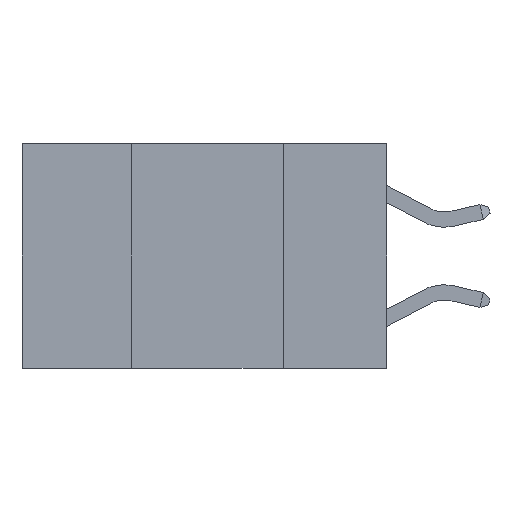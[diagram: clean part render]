
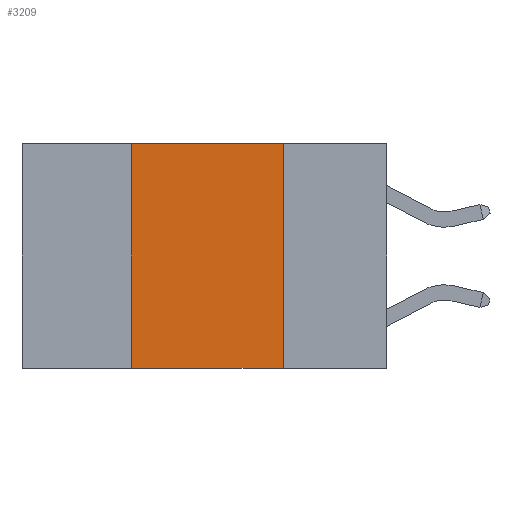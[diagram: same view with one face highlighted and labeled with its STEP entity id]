
A CAD part, left-side view. The second image highlights one B-rep face of the part: STEP entity #3209.
In plain terms, the highlighted planar face has unit normal (-1, 0, 0).
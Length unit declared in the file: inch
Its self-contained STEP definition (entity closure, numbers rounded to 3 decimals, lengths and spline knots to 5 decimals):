
#178 = LINE ( 'NONE', #4160, #14691 ) ;
#516 = EDGE_CURVE ( 'NONE', #11932, #4437, #6694, .T. ) ;
#741 = CARTESIAN_POINT ( 'NONE',  ( 0., 0.17, 0. ) ) ;
#879 = LINE ( 'NONE', #4568, #3562 ) ;
#1176 = CARTESIAN_POINT ( 'NONE',  ( 0., 0.42, 0. ) ) ;
#2120 = DIRECTION ( 'NONE',  ( 0., -1., 0. ) ) ;
#2227 = EDGE_CURVE ( 'NONE', #11945, #11932, #8086, .T. ) ;
#2247 = EDGE_CURVE ( 'NONE', #4437, #12415, #879, .T. ) ;
#2330 = EDGE_CURVE ( 'NONE', #11945, #12415, #178, .T. ) ;
#2618 = DIRECTION ( 'NONE',  ( 0., 0., 1. ) ) ;
#3209 = ADVANCED_FACE ( 'NONE', ( #7870 ), #11098, .F. ) ;
#3328 = CARTESIAN_POINT ( 'NONE',  ( 0., 0.17, -0.37 ) ) ;
#3562 = VECTOR ( 'NONE', #4903, 39.37008 ) ;
#4160 = CARTESIAN_POINT ( 'NONE',  ( 0., 0.6, -0.37 ) ) ;
#4239 = DIRECTION ( 'NONE',  ( 1., 0., 0. ) ) ;
#4437 = VERTEX_POINT ( 'NONE', #741 ) ;
#4568 = CARTESIAN_POINT ( 'NONE',  ( 0., 0.17, 0. ) ) ;
#4903 = DIRECTION ( 'NONE',  ( 0., 0., -1. ) ) ;
#4914 = ORIENTED_EDGE ( 'NONE', *, *, #2330, .T. ) ;
#6694 = LINE ( 'NONE', #12723, #9384 ) ;
#7870 = FACE_OUTER_BOUND ( 'NONE', #8855, .T. ) ;
#7889 = CARTESIAN_POINT ( 'NONE',  ( 0., 0.42, 0. ) ) ;
#8086 = LINE ( 'NONE', #7889, #10042 ) ;
#8855 = EDGE_LOOP ( 'NONE', ( #9961, #10309, #13708, #4914 ) ) ;
#9129 = DIRECTION ( 'NONE',  ( 0., -1., 0. ) ) ;
#9384 = VECTOR ( 'NONE', #9129, 39.37008 ) ;
#9961 = ORIENTED_EDGE ( 'NONE', *, *, #2247, .F. ) ;
#10042 = VECTOR ( 'NONE', #2618, 39.37008 ) ;
#10309 = ORIENTED_EDGE ( 'NONE', *, *, #516, .F. ) ;
#10359 = CARTESIAN_POINT ( 'NONE',  ( 0., 0.42, -0.37 ) ) ;
#11098 = PLANE ( 'NONE',  #13972 ) ;
#11932 = VERTEX_POINT ( 'NONE', #1176 ) ;
#11945 = VERTEX_POINT ( 'NONE', #10359 ) ;
#12248 = DIRECTION ( 'NONE',  ( 0., 0., -1. ) ) ;
#12415 = VERTEX_POINT ( 'NONE', #3328 ) ;
#12723 = CARTESIAN_POINT ( 'NONE',  ( 0., 0.6, 0. ) ) ;
#13708 = ORIENTED_EDGE ( 'NONE', *, *, #2227, .F. ) ;
#13972 = AXIS2_PLACEMENT_3D ( 'NONE', #14510, #4239, #12248 ) ;
#14510 = CARTESIAN_POINT ( 'NONE',  ( 0., 0.6, 0. ) ) ;
#14691 = VECTOR ( 'NONE', #2120, 39.37008 ) ;
